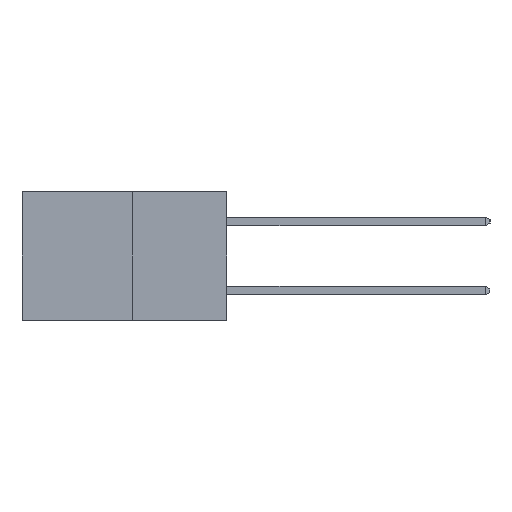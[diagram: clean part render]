
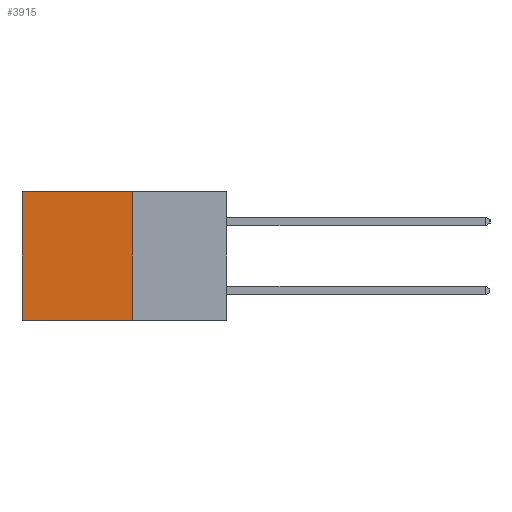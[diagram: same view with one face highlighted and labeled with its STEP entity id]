
A CAD part, left-side view. The second image highlights one B-rep face of the part: STEP entity #3915.
In plain terms, the highlighted planar face has unit normal (-1, 0, 0).
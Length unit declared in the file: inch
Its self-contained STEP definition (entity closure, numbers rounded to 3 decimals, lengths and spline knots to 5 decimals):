
#275 = ORIENTED_EDGE ( 'NONE', *, *, #3019, .T. ) ;
#331 = VERTEX_POINT ( 'NONE', #3064 ) ;
#680 = CARTESIAN_POINT ( 'NONE',  ( 0.277, 0.27, 0. ) ) ;
#771 = VERTEX_POINT ( 'NONE', #1016 ) ;
#931 = DIRECTION ( 'NONE',  ( 1., 0., 0. ) ) ;
#1016 = CARTESIAN_POINT ( 'NONE',  ( 0.277, 0.59, 0. ) ) ;
#1112 = EDGE_CURVE ( 'NONE', #1160, #2923, #3671, .T. ) ;
#1160 = VERTEX_POINT ( 'NONE', #680 ) ;
#1174 = LINE ( 'NONE', #8759, #6622 ) ;
#1236 = DIRECTION ( 'NONE',  ( 0., 0., -1. ) ) ;
#1311 = ORIENTED_EDGE ( 'NONE', *, *, #6307, .F. ) ;
#1351 = EDGE_LOOP ( 'NONE', ( #275, #1311, #7422, #3868 ) ) ;
#1768 = CARTESIAN_POINT ( 'NONE',  ( 0.277, 0.27, 0. ) ) ;
#2262 = CARTESIAN_POINT ( 'NONE',  ( 0.277, 0.27, -0.37 ) ) ;
#2740 = AXIS2_PLACEMENT_3D ( 'NONE', #5489, #931, #6183 ) ;
#2923 = VERTEX_POINT ( 'NONE', #4591 ) ;
#3019 = EDGE_CURVE ( 'NONE', #771, #331, #3883, .T. ) ;
#3064 = CARTESIAN_POINT ( 'NONE',  ( 0.277, 0.59, -0.37 ) ) ;
#3671 = LINE ( 'NONE', #2262, #5394 ) ;
#3858 = VECTOR ( 'NONE', #4837, 39.37008 ) ;
#3868 = ORIENTED_EDGE ( 'NONE', *, *, #6395, .T. ) ;
#3883 = LINE ( 'NONE', #4927, #9097 ) ;
#3915 = ADVANCED_FACE ( 'NONE', ( #4680 ), #6153, .F. ) ;
#4591 = CARTESIAN_POINT ( 'NONE',  ( 0.277, 0.27, -0.37 ) ) ;
#4680 = FACE_OUTER_BOUND ( 'NONE', #1351, .T. ) ;
#4742 = DIRECTION ( 'NONE',  ( 0., 1., 0. ) ) ;
#4837 = DIRECTION ( 'NONE',  ( 0., 1., 0. ) ) ;
#4927 = CARTESIAN_POINT ( 'NONE',  ( 0.277, 0.59, -0.37 ) ) ;
#5394 = VECTOR ( 'NONE', #1236, 39.37008 ) ;
#5489 = CARTESIAN_POINT ( 'NONE',  ( 0.277, 0.27, -0.37 ) ) ;
#5566 = LINE ( 'NONE', #1768, #3858 ) ;
#6153 = PLANE ( 'NONE',  #2740 ) ;
#6183 = DIRECTION ( 'NONE',  ( 0., 0., -1. ) ) ;
#6307 = EDGE_CURVE ( 'NONE', #2923, #331, #1174, .T. ) ;
#6395 = EDGE_CURVE ( 'NONE', #1160, #771, #5566, .T. ) ;
#6622 = VECTOR ( 'NONE', #4742, 39.37008 ) ;
#7010 = DIRECTION ( 'NONE',  ( 0., 0., -1. ) ) ;
#7422 = ORIENTED_EDGE ( 'NONE', *, *, #1112, .F. ) ;
#8759 = CARTESIAN_POINT ( 'NONE',  ( 0.277, 0.27, -0.37 ) ) ;
#9097 = VECTOR ( 'NONE', #7010, 39.37008 ) ;
